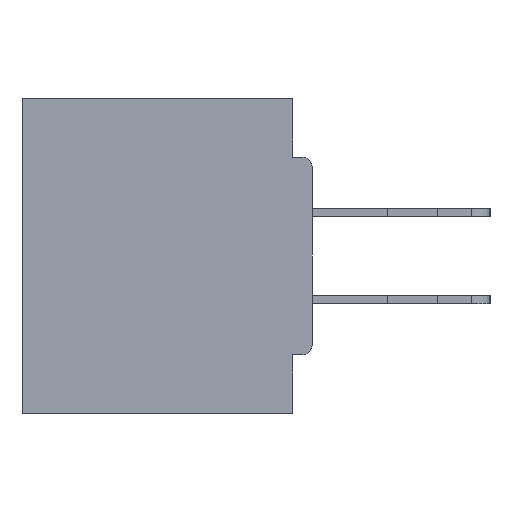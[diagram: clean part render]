
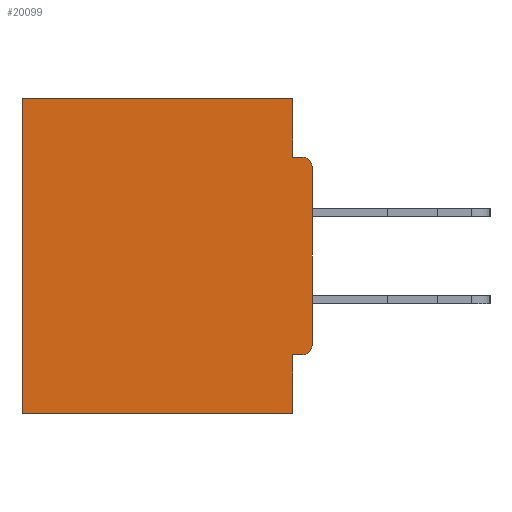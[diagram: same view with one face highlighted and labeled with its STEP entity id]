
A CAD part, left-side view. The second image highlights one B-rep face of the part: STEP entity #20099.
In plain terms, the highlighted planar face has unit normal (-1, 0, 0).
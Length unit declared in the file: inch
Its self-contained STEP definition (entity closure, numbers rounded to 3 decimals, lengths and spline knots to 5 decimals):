
#1 = ORIENTED_EDGE ( 'NONE', *, *, #6541, .T. ) ;
#95 = EDGE_CURVE ( 'NONE', #31311, #17192, #14440, .T. ) ;
#490 = AXIS2_PLACEMENT_3D ( 'NONE', #17145, #4444, #24026 ) ;
#1693 = LINE ( 'NONE', #21664, #28269 ) ;
#2488 = EDGE_CURVE ( 'NONE', #10467, #35367, #32755, .T. ) ;
#2535 = EDGE_LOOP ( 'NONE', ( #18963, #15384, #3819, #1, #30830, #23860, #16740, #31213, #40618, #17794 ) ) ;
#2880 = LINE ( 'NONE', #31014, #3356 ) ;
#2893 = DIRECTION ( 'NONE',  ( 0., 1., 0. ) ) ;
#3356 = VECTOR ( 'NONE', #21917, 39.37008 ) ;
#3445 = DIRECTION ( 'NONE',  ( -1., 0., 0. ) ) ;
#3819 = ORIENTED_EDGE ( 'NONE', *, *, #31607, .F. ) ;
#3908 = AXIS2_PLACEMENT_3D ( 'NONE', #38510, #3445, #22080 ) ;
#4444 = DIRECTION ( 'NONE',  ( 1., 0., 0. ) ) ;
#5378 = AXIS2_PLACEMENT_3D ( 'NONE', #18723, #38135, #6546 ) ;
#5558 = DIRECTION ( 'NONE',  ( 0., 0., -1. ) ) ;
#5967 = VECTOR ( 'NONE', #2893, 39.37008 ) ;
#6541 = EDGE_CURVE ( 'NONE', #17835, #30700, #2880, .T. ) ;
#6546 = DIRECTION ( 'NONE',  ( 0., 0., -1. ) ) ;
#6569 = VECTOR ( 'NONE', #29250, 39.37008 ) ;
#7422 = EDGE_CURVE ( 'NONE', #37262, #8360, #36825, .T. ) ;
#7635 = CARTESIAN_POINT ( 'NONE',  ( 0.298, 0.031, -0.5 ) ) ;
#7768 = DIRECTION ( 'NONE',  ( 0., 1., 0. ) ) ;
#8360 = VERTEX_POINT ( 'NONE', #18117 ) ;
#8867 = DIRECTION ( 'NONE',  ( 0., 0., -1. ) ) ;
#10467 = VERTEX_POINT ( 'NONE', #38083 ) ;
#11061 = LINE ( 'NONE', #7635, #27633 ) ;
#11514 = CARTESIAN_POINT ( 'NONE',  ( 0.298, 0.46, -0.5 ) ) ;
#11899 = CARTESIAN_POINT ( 'NONE',  ( 0.298, 0.46, 0. ) ) ;
#13331 = FACE_OUTER_BOUND ( 'NONE', #2535, .T. ) ;
#13444 = VERTEX_POINT ( 'NONE', #22840 ) ;
#14440 = LINE ( 'NONE', #22927, #5967 ) ;
#15312 = CARTESIAN_POINT ( 'NONE',  ( 0.298, 0., -0.0935 ) ) ;
#15384 = ORIENTED_EDGE ( 'NONE', *, *, #7422, .F. ) ;
#16740 = ORIENTED_EDGE ( 'NONE', *, *, #38362, .F. ) ;
#17145 = CARTESIAN_POINT ( 'NONE',  ( 0.298, 0., 0. ) ) ;
#17192 = VERTEX_POINT ( 'NONE', #11514 ) ;
#17346 = EDGE_CURVE ( 'NONE', #10467, #40443, #21080, .T. ) ;
#17794 = ORIENTED_EDGE ( 'NONE', *, *, #23533, .F. ) ;
#17835 = VERTEX_POINT ( 'NONE', #28473 ) ;
#18117 = CARTESIAN_POINT ( 'NONE',  ( 0.298, 0.015, -0.0935 ) ) ;
#18723 = CARTESIAN_POINT ( 'NONE',  ( 0.298, 0.015, -0.1085 ) ) ;
#18751 = VECTOR ( 'NONE', #7768, 39.37008 ) ;
#18963 = ORIENTED_EDGE ( 'NONE', *, *, #22762, .T. ) ;
#20099 = ADVANCED_FACE ( 'NONE', ( #13331 ), #29901, .F. ) ;
#20656 = CIRCLE ( 'NONE', #5378, 0.015 ) ;
#21080 = CIRCLE ( 'NONE', #3908, 0.015 ) ;
#21664 = CARTESIAN_POINT ( 'NONE',  ( 0.298, 0.46, 0. ) ) ;
#21917 = DIRECTION ( 'NONE',  ( 0., 1., 0. ) ) ;
#22080 = DIRECTION ( 'NONE',  ( 0., 0., -1. ) ) ;
#22315 = VECTOR ( 'NONE', #8867, 39.37008 ) ;
#22762 = EDGE_CURVE ( 'NONE', #13444, #8360, #20656, .T. ) ;
#22840 = CARTESIAN_POINT ( 'NONE',  ( 0.298, 0., -0.1085 ) ) ;
#22844 = VECTOR ( 'NONE', #37667, 39.37008 ) ;
#22927 = CARTESIAN_POINT ( 'NONE',  ( 0.298, 0., -0.5 ) ) ;
#23533 = EDGE_CURVE ( 'NONE', #13444, #40443, #33625, .T. ) ;
#23860 = ORIENTED_EDGE ( 'NONE', *, *, #95, .F. ) ;
#24026 = DIRECTION ( 'NONE',  ( 0., 0., -1. ) ) ;
#26947 = CARTESIAN_POINT ( 'NONE',  ( 0.298, 0., -0.4065 ) ) ;
#27633 = VECTOR ( 'NONE', #29601, 39.37008 ) ;
#28269 = VECTOR ( 'NONE', #5558, 39.37008 ) ;
#28473 = CARTESIAN_POINT ( 'NONE',  ( 0.298, 0.031, 0. ) ) ;
#28794 = CARTESIAN_POINT ( 'NONE',  ( 0.298, 0.031, -0.5 ) ) ;
#29250 = DIRECTION ( 'NONE',  ( 0., 0., -1. ) ) ;
#29601 = DIRECTION ( 'NONE',  ( 0., 0., -1. ) ) ;
#29901 = PLANE ( 'NONE',  #490 ) ;
#30700 = VERTEX_POINT ( 'NONE', #11899 ) ;
#30830 = ORIENTED_EDGE ( 'NONE', *, *, #38996, .T. ) ;
#31014 = CARTESIAN_POINT ( 'NONE',  ( 0.298, 0., 0. ) ) ;
#31213 = ORIENTED_EDGE ( 'NONE', *, *, #2488, .F. ) ;
#31311 = VERTEX_POINT ( 'NONE', #28794 ) ;
#31607 = EDGE_CURVE ( 'NONE', #17835, #37262, #11061, .T. ) ;
#32755 = LINE ( 'NONE', #26947, #18751 ) ;
#33106 = CARTESIAN_POINT ( 'NONE',  ( 0.298, 0.031, -0.4065 ) ) ;
#33625 = LINE ( 'NONE', #38857, #6569 ) ;
#35367 = VERTEX_POINT ( 'NONE', #33106 ) ;
#35890 = CARTESIAN_POINT ( 'NONE',  ( 0.298, 0., -0.3915 ) ) ;
#36825 = LINE ( 'NONE', #15312, #22844 ) ;
#37262 = VERTEX_POINT ( 'NONE', #39296 ) ;
#37667 = DIRECTION ( 'NONE',  ( 0., -1., 0. ) ) ;
#38083 = CARTESIAN_POINT ( 'NONE',  ( 0.298, 0.015, -0.4065 ) ) ;
#38135 = DIRECTION ( 'NONE',  ( -1., 0., 0. ) ) ;
#38362 = EDGE_CURVE ( 'NONE', #35367, #31311, #39730, .T. ) ;
#38510 = CARTESIAN_POINT ( 'NONE',  ( 0.298, 0.015, -0.3915 ) ) ;
#38857 = CARTESIAN_POINT ( 'NONE',  ( 0.298, 0., 0. ) ) ;
#38996 = EDGE_CURVE ( 'NONE', #30700, #17192, #1693, .T. ) ;
#39296 = CARTESIAN_POINT ( 'NONE',  ( 0.298, 0.031, -0.0935 ) ) ;
#39730 = LINE ( 'NONE', #41387, #22315 ) ;
#40443 = VERTEX_POINT ( 'NONE', #35890 ) ;
#40618 = ORIENTED_EDGE ( 'NONE', *, *, #17346, .T. ) ;
#41387 = CARTESIAN_POINT ( 'NONE',  ( 0.298, 0.031, -0.5 ) ) ;
